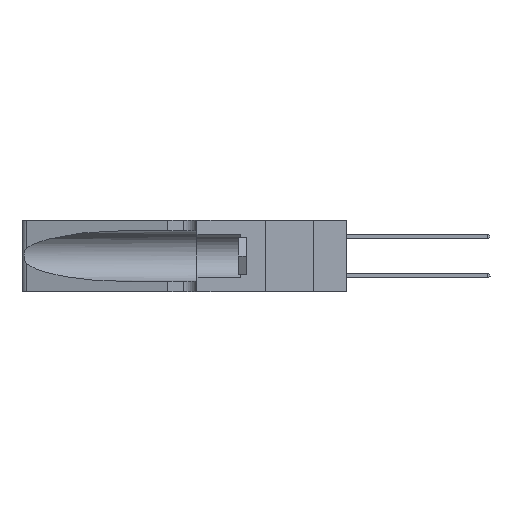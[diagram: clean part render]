
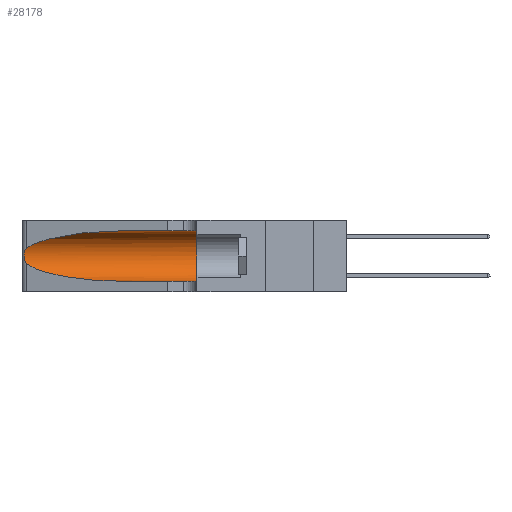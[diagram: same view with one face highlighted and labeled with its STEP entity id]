
A CAD part, left-side view. The second image highlights one B-rep face of the part: STEP entity #28178.
In plain terms, the highlighted cylindrical face has radius 3.308 mm (diameter 6.617 mm), a partial arc.
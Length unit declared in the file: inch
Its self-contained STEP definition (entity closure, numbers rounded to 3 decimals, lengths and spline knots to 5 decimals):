
#15 = CARTESIAN_POINT ( 'NONE',  ( 0.1305, 0.72297, 0.05475 ) ) ;
#72 = LINE ( 'NONE', #8746, #12672 ) ;
#467 = CARTESIAN_POINT ( 'NONE',  ( 0.25487, 1.22718, 0.14631 ) ) ;
#847 = CARTESIAN_POINT ( 'NONE',  ( 0.26075, 1.23896, 0.19203 ) ) ;
#2251 = EDGE_CURVE ( 'NONE', #11137, #31539, #8108, .T. ) ;
#3296 = ORIENTED_EDGE ( 'NONE', *, *, #10833, .T. ) ;
#3418 = CARTESIAN_POINT ( 'NONE',  ( 0.25639, 1.23184, 0.21858 ) ) ;
#3535 = CARTESIAN_POINT ( 'NONE',  ( 0.26075, 1.23896, 0.178 ) ) ;
#3622 = CARTESIAN_POINT ( 'NONE',  ( 0.1305, 0.72297, 0.05475 ) ) ;
#5356 = CARTESIAN_POINT ( 'NONE',  ( 0.2373, 1.15595, 0.28018 ) ) ;
#5610 = CARTESIAN_POINT ( 'NONE',  ( 0.18966, 0.96281, 0.31525 ) ) ;
#5923 = AXIS2_PLACEMENT_3D ( 'NONE', #19125, #32688, #19483 ) ;
#6059 = DIRECTION ( 'NONE',  ( 0., -1., 0. ) ) ;
#6223 = CARTESIAN_POINT ( 'NONE',  ( 0.25856, 1.23593, 0.16098 ) ) ;
#7683 = DIRECTION ( 'NONE',  ( 0., 0., 1. ) ) ;
#8038 = CARTESIAN_POINT ( 'NONE',  ( 0.25487, 1.22718, 0.22369 ) ) ;
#8108 =( BOUNDED_CURVE ( )  B_SPLINE_CURVE ( 3, ( #467, #11256, #12182, #3622 ),
 .UNSPECIFIED., .F., .T. ) 
 B_SPLINE_CURVE_WITH_KNOTS ( ( 4, 4 ),
 ( 3.44316, 4.71239 ),
 .UNSPECIFIED. ) 
 CURVE ( )  GEOMETRIC_REPRESENTATION_ITEM ( )  RATIONAL_B_SPLINE_CURVE ( ( 1., 0.87, 0.87, 1. ) ) 
 REPRESENTATION_ITEM ( '' )  );
#8746 = CARTESIAN_POINT ( 'NONE',  ( 0.1305, 1.61858, 0.31525 ) ) ;
#8791 = CARTESIAN_POINT ( 'NONE',  ( 0.26018, 1.23835, 0.19895 ) ) ;
#10008 = ORIENTED_EDGE ( 'NONE', *, *, #2251, .T. ) ;
#10118 = ORIENTED_EDGE ( 'NONE', *, *, #32409, .F. ) ;
#10147 = ORIENTED_EDGE ( 'NONE', *, *, #25653, .F. ) ;
#10168 = VECTOR ( 'NONE', #29663, 39.37008 ) ;
#10833 = EDGE_CURVE ( 'NONE', #31539, #15787, #12317, .T. ) ;
#11137 = VERTEX_POINT ( 'NONE', #16292 ) ;
#11256 = CARTESIAN_POINT ( 'NONE',  ( 0.2373, 1.15595, 0.08982 ) ) ;
#11637 = CARTESIAN_POINT ( 'NONE',  ( 0.1305, 0.72297, 0.31525 ) ) ;
#11708 = FACE_OUTER_BOUND ( 'NONE', #12259, .T. ) ;
#12182 = CARTESIAN_POINT ( 'NONE',  ( 0.18966, 0.96281, 0.05475 ) ) ;
#12259 = EDGE_LOOP ( 'NONE', ( #25711, #33177, #10008, #3296, #10147, #10118 ) ) ;
#12317 = LINE ( 'NONE', #24567, #10168 ) ;
#12672 = VECTOR ( 'NONE', #6059, 39.37008 ) ;
#13057 = AXIS2_PLACEMENT_3D ( 'NONE', #34365, #15561, #7683 ) ;
#13346 = CYLINDRICAL_SURFACE ( 'NONE', #5923, 0.13025 ) ;
#15561 = DIRECTION ( 'NONE',  ( 0., 1., 0. ) ) ;
#15787 = VERTEX_POINT ( 'NONE', #19782 ) ;
#16292 = CARTESIAN_POINT ( 'NONE',  ( 0.25487, 1.22718, 0.14631 ) ) ;
#17145 = VERTEX_POINT ( 'NONE', #26203 ) ;
#17565 = CARTESIAN_POINT ( 'NONE',  ( 0.25487, 1.22718, 0.14631 ) ) ;
#19125 = CARTESIAN_POINT ( 'NONE',  ( 0.1305, 1.61858, 0.185 ) ) ;
#19266 = EDGE_CURVE ( 'NONE', #23537, #31695, #24516, .T. ) ;
#19316 = CARTESIAN_POINT ( 'NONE',  ( 0.25787, 1.23484, 0.2124 ) ) ;
#19483 = DIRECTION ( 'NONE',  ( 0., 0., -1. ) ) ;
#19659 = CARTESIAN_POINT ( 'NONE',  ( 0.25555, 1.22993, 0.14849 ) ) ;
#19782 = CARTESIAN_POINT ( 'NONE',  ( 0.1305, 0.35, 0.05475 ) ) ;
#21213 = CIRCLE ( 'NONE', #13057, 0.13025 ) ;
#22251 = CARTESIAN_POINT ( 'NONE',  ( 0.26017, 1.23833, 0.17102 ) ) ;
#23537 = VERTEX_POINT ( 'NONE', #30387 ) ;
#24516 =( BOUNDED_CURVE ( )  B_SPLINE_CURVE ( 3, ( #11637, #5610, #5356, #8038 ),
 .UNSPECIFIED., .F., .F. ) 
 B_SPLINE_CURVE_WITH_KNOTS ( ( 4, 4 ),
 ( 1.5708, 2.84003 ),
 .UNSPECIFIED. ) 
 CURVE ( )  GEOMETRIC_REPRESENTATION_ITEM ( )  RATIONAL_B_SPLINE_CURVE ( ( 1., 0.87, 0.87, 1. ) ) 
 REPRESENTATION_ITEM ( '' )  );
#24567 = CARTESIAN_POINT ( 'NONE',  ( 0.1305, 1.61858, 0.05475 ) ) ;
#24826 = CARTESIAN_POINT ( 'NONE',  ( 0.25854, 1.2359, 0.20912 ) ) ;
#24932 = CARTESIAN_POINT ( 'NONE',  ( 0.25789, 1.23486, 0.15765 ) ) ;
#25158 = CARTESIAN_POINT ( 'NONE',  ( 0.25487, 1.22718, 0.22369 ) ) ;
#25653 = EDGE_CURVE ( 'NONE', #17145, #15787, #21213, .T. ) ;
#25711 = ORIENTED_EDGE ( 'NONE', *, *, #19266, .T. ) ;
#26203 = CARTESIAN_POINT ( 'NONE',  ( 0.1305, 0.35, 0.31525 ) ) ;
#27039 = B_SPLINE_CURVE_WITH_KNOTS ( 'NONE', 3,
 ( #25158, #32749, #3418, #19316, #24826, #8791, #847, #3535, #22251, #6223, #24932, #27590, #19659, #17565 ),
 .UNSPECIFIED., .F., .F.,
 ( 4, 2, 2, 2, 2, 2, 4 ),
 ( 0., 0.00027, 0.00053, 0.00107, 0.0016, 0.00187, 0.00214 ),
 .UNSPECIFIED. ) ;
#27468 = CARTESIAN_POINT ( 'NONE',  ( 0.25487, 1.22718, 0.22369 ) ) ;
#27590 = CARTESIAN_POINT ( 'NONE',  ( 0.25639, 1.23186, 0.15144 ) ) ;
#28178 = ADVANCED_FACE ( 'NONE', ( #11708 ), #13346, .F. ) ;
#29663 = DIRECTION ( 'NONE',  ( 0., -1., 0. ) ) ;
#30387 = CARTESIAN_POINT ( 'NONE',  ( 0.1305, 0.72297, 0.31525 ) ) ;
#31539 = VERTEX_POINT ( 'NONE', #15 ) ;
#31695 = VERTEX_POINT ( 'NONE', #27468 ) ;
#31786 = EDGE_CURVE ( 'NONE', #31695, #11137, #27039, .T. ) ;
#32409 = EDGE_CURVE ( 'NONE', #23537, #17145, #72, .T. ) ;
#32688 = DIRECTION ( 'NONE',  ( 0., -1., 0. ) ) ;
#32749 = CARTESIAN_POINT ( 'NONE',  ( 0.25555, 1.22994, 0.2215 ) ) ;
#33177 = ORIENTED_EDGE ( 'NONE', *, *, #31786, .T. ) ;
#34365 = CARTESIAN_POINT ( 'NONE',  ( 0.1305, 0.35, 0.185 ) ) ;
